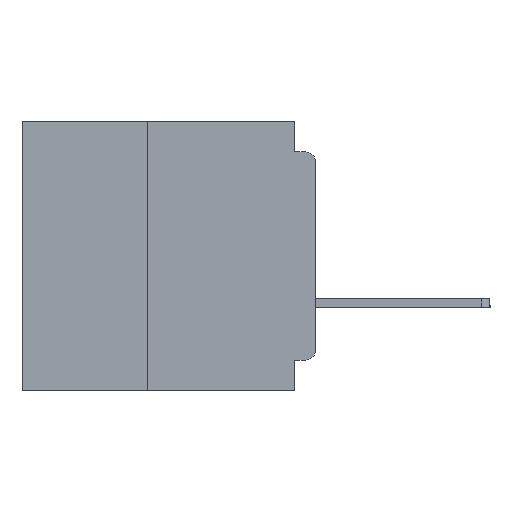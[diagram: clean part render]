
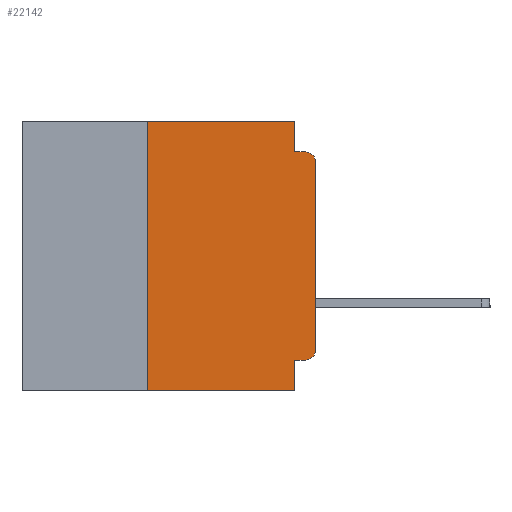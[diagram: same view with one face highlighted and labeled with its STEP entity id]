
A CAD part, left-side view. The second image highlights one B-rep face of the part: STEP entity #22142.
In plain terms, the highlighted planar face has unit normal (-1, 0, 0).
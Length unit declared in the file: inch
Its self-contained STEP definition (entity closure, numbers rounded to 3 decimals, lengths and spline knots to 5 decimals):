
#371 = VERTEX_POINT ( 'NONE', #17752 ) ;
#1442 = CARTESIAN_POINT ( 'NONE',  ( 0., 0.015, -0.06 ) ) ;
#1607 = EDGE_CURVE ( 'NONE', #23963, #28432, #34634, .T. ) ;
#3145 = CARTESIAN_POINT ( 'NONE',  ( 0., 0., 0. ) ) ;
#3231 = CARTESIAN_POINT ( 'NONE',  ( 0., 0.031, 0. ) ) ;
#3806 = LINE ( 'NONE', #5877, #12927 ) ;
#3970 = EDGE_CURVE ( 'NONE', #23963, #14306, #6483, .T. ) ;
#4717 = ORIENTED_EDGE ( 'NONE', *, *, #3970, .F. ) ;
#4941 = DIRECTION ( 'NONE',  ( 0., 0., -1. ) ) ;
#5154 = EDGE_CURVE ( 'NONE', #20879, #27402, #37935, .T. ) ;
#5262 = ORIENTED_EDGE ( 'NONE', *, *, #5154, .T. ) ;
#5407 = VERTEX_POINT ( 'NONE', #12428 ) ;
#5877 = CARTESIAN_POINT ( 'NONE',  ( 0., 0., -0.355 ) ) ;
#6276 = EDGE_CURVE ( 'NONE', #42211, #11621, #9995, .T. ) ;
#6483 = LINE ( 'NONE', #21527, #41785 ) ;
#7385 = VECTOR ( 'NONE', #28579, 39.37008 ) ;
#7793 = LINE ( 'NONE', #3145, #30779 ) ;
#7796 = DIRECTION ( 'NONE',  ( 0., 0., 1. ) ) ;
#7877 = VECTOR ( 'NONE', #40936, 39.37008 ) ;
#9650 = CARTESIAN_POINT ( 'NONE',  ( 0., 0.031, -0.045 ) ) ;
#9995 = LINE ( 'NONE', #3231, #7877 ) ;
#10494 = ORIENTED_EDGE ( 'NONE', *, *, #34279, .F. ) ;
#10984 = AXIS2_PLACEMENT_3D ( 'NONE', #34857, #14418, #38313 ) ;
#11201 = CARTESIAN_POINT ( 'NONE',  ( 0., 0.015, -0.355 ) ) ;
#11380 = DIRECTION ( 'NONE',  ( 0., 0., -1. ) ) ;
#11621 = VERTEX_POINT ( 'NONE', #9650 ) ;
#11744 = CARTESIAN_POINT ( 'NONE',  ( 0., 0.25, -0.4 ) ) ;
#11876 = VECTOR ( 'NONE', #33560, 39.37008 ) ;
#12428 = CARTESIAN_POINT ( 'NONE',  ( 0., 0.015, -0.045 ) ) ;
#12927 = VECTOR ( 'NONE', #22951, 39.37008 ) ;
#13222 = AXIS2_PLACEMENT_3D ( 'NONE', #14686, #31871, #11380 ) ;
#14274 = EDGE_LOOP ( 'NONE', ( #44164, #22435, #18844, #21090, #10494, #4717, #41273, #22394, #29601, #5262 ) ) ;
#14306 = VERTEX_POINT ( 'NONE', #25025 ) ;
#14364 = EDGE_CURVE ( 'NONE', #20400, #5407, #40557, .T. ) ;
#14418 = DIRECTION ( 'NONE',  ( -1., 0., 0. ) ) ;
#14686 = CARTESIAN_POINT ( 'NONE',  ( 0., 0.437, 0. ) ) ;
#15786 = EDGE_CURVE ( 'NONE', #27402, #20400, #7793, .T. ) ;
#16280 = FACE_OUTER_BOUND ( 'NONE', #14274, .T. ) ;
#16943 = DIRECTION ( 'NONE',  ( 0., 0., 1. ) ) ;
#17091 = DIRECTION ( 'NONE',  ( 0., 0., -1. ) ) ;
#17752 = CARTESIAN_POINT ( 'NONE',  ( 0., 0.031, -0.355 ) ) ;
#18510 = VECTOR ( 'NONE', #43345, 39.37008 ) ;
#18844 = ORIENTED_EDGE ( 'NONE', *, *, #44115, .F. ) ;
#20400 = VERTEX_POINT ( 'NONE', #25744 ) ;
#20879 = VERTEX_POINT ( 'NONE', #11201 ) ;
#21090 = ORIENTED_EDGE ( 'NONE', *, *, #6276, .F. ) ;
#21527 = CARTESIAN_POINT ( 'NONE',  ( 0., 0.25, -0.4 ) ) ;
#21554 = PLANE ( 'NONE',  #13222 ) ;
#22142 = ADVANCED_FACE ( 'NONE', ( #16280 ), #21554, .F. ) ;
#22394 = ORIENTED_EDGE ( 'NONE', *, *, #43783, .F. ) ;
#22435 = ORIENTED_EDGE ( 'NONE', *, *, #14364, .T. ) ;
#22951 = DIRECTION ( 'NONE',  ( 0., 1., 0. ) ) ;
#23963 = VERTEX_POINT ( 'NONE', #11744 ) ;
#25025 = CARTESIAN_POINT ( 'NONE',  ( 0., 0.25, 0. ) ) ;
#25161 = CARTESIAN_POINT ( 'NONE',  ( 0., 0.437, -0.4 ) ) ;
#25462 = DIRECTION ( 'NONE',  ( -1., 0., 0. ) ) ;
#25545 = CARTESIAN_POINT ( 'NONE',  ( 0., 0., -0.34 ) ) ;
#25744 = CARTESIAN_POINT ( 'NONE',  ( 0., 0., -0.06 ) ) ;
#26190 = CARTESIAN_POINT ( 'NONE',  ( 0., 0., -0.045 ) ) ;
#27402 = VERTEX_POINT ( 'NONE', #25545 ) ;
#28103 = EDGE_CURVE ( 'NONE', #20879, #371, #3806, .T. ) ;
#28432 = VERTEX_POINT ( 'NONE', #38301 ) ;
#28579 = DIRECTION ( 'NONE',  ( 0., -1., 0. ) ) ;
#28696 = LINE ( 'NONE', #26190, #18510 ) ;
#29601 = ORIENTED_EDGE ( 'NONE', *, *, #28103, .F. ) ;
#30118 = CARTESIAN_POINT ( 'NONE',  ( 0., 0.437, 0. ) ) ;
#30779 = VECTOR ( 'NONE', #16943, 39.37008 ) ;
#31871 = DIRECTION ( 'NONE',  ( 1., 0., 0. ) ) ;
#33095 = CARTESIAN_POINT ( 'NONE',  ( 0., 0.031, 0. ) ) ;
#33535 = LINE ( 'NONE', #37657, #42622 ) ;
#33560 = DIRECTION ( 'NONE',  ( 0., -1., 0. ) ) ;
#34279 = EDGE_CURVE ( 'NONE', #14306, #42211, #39143, .T. ) ;
#34634 = LINE ( 'NONE', #25161, #7385 ) ;
#34782 = AXIS2_PLACEMENT_3D ( 'NONE', #1442, #25462, #4941 ) ;
#34857 = CARTESIAN_POINT ( 'NONE',  ( 0., 0.015, -0.34 ) ) ;
#37657 = CARTESIAN_POINT ( 'NONE',  ( 0., 0.031, -0.4 ) ) ;
#37935 = CIRCLE ( 'NONE', #10984, 0.015 ) ;
#38301 = CARTESIAN_POINT ( 'NONE',  ( 0., 0.031, -0.4 ) ) ;
#38313 = DIRECTION ( 'NONE',  ( 0., 0., -1. ) ) ;
#39143 = LINE ( 'NONE', #30118, #11876 ) ;
#40557 = CIRCLE ( 'NONE', #34782, 0.015 ) ;
#40936 = DIRECTION ( 'NONE',  ( 0., 0., -1. ) ) ;
#41273 = ORIENTED_EDGE ( 'NONE', *, *, #1607, .T. ) ;
#41785 = VECTOR ( 'NONE', #7796, 39.37008 ) ;
#42211 = VERTEX_POINT ( 'NONE', #33095 ) ;
#42622 = VECTOR ( 'NONE', #17091, 39.37008 ) ;
#43345 = DIRECTION ( 'NONE',  ( 0., -1., 0. ) ) ;
#43783 = EDGE_CURVE ( 'NONE', #371, #28432, #33535, .T. ) ;
#44115 = EDGE_CURVE ( 'NONE', #11621, #5407, #28696, .T. ) ;
#44164 = ORIENTED_EDGE ( 'NONE', *, *, #15786, .T. ) ;
